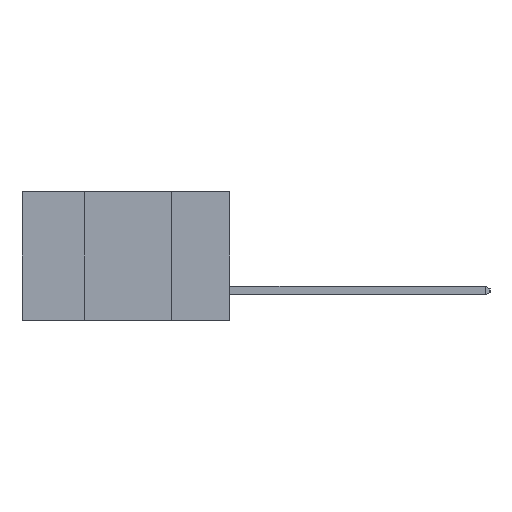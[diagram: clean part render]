
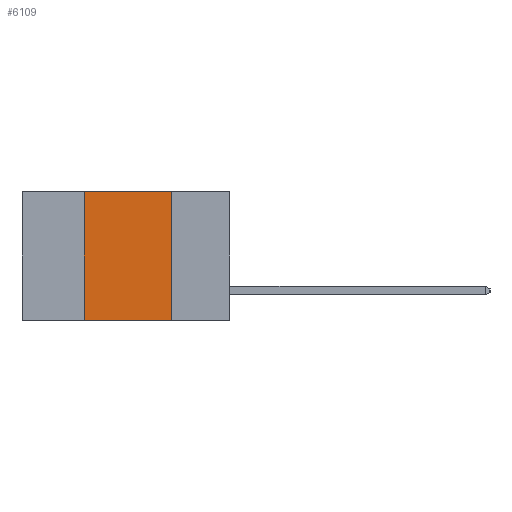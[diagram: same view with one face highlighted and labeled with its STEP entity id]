
A CAD part, left-side view. The second image highlights one B-rep face of the part: STEP entity #6109.
In plain terms, the highlighted planar face has unit normal (-1, 0, 0).
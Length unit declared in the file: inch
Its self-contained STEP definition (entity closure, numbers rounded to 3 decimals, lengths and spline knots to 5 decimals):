
#639 = CARTESIAN_POINT ( 'NONE',  ( 0., 0.6, -0.37 ) ) ;
#677 = LINE ( 'NONE', #12939, #9490 ) ;
#1038 = CARTESIAN_POINT ( 'NONE',  ( 0., 0.17, -0.37 ) ) ;
#1092 = LINE ( 'NONE', #10749, #21576 ) ;
#2657 = EDGE_CURVE ( 'NONE', #11655, #3269, #677, .T. ) ;
#3269 = VERTEX_POINT ( 'NONE', #16123 ) ;
#3472 = EDGE_CURVE ( 'NONE', #22373, #11655, #1092, .T. ) ;
#6109 = ADVANCED_FACE ( 'NONE', ( #21438 ), #7681, .F. ) ;
#6557 = VERTEX_POINT ( 'NONE', #1038 ) ;
#6902 = VECTOR ( 'NONE', #10671, 39.37008 ) ;
#7468 = ORIENTED_EDGE ( 'NONE', *, *, #3472, .F. ) ;
#7681 = PLANE ( 'NONE',  #22489 ) ;
#7974 = DIRECTION ( 'NONE',  ( 0., 0., 1. ) ) ;
#9490 = VECTOR ( 'NONE', #12769, 39.37008 ) ;
#9627 = DIRECTION ( 'NONE',  ( 0., 0., -1. ) ) ;
#10671 = DIRECTION ( 'NONE',  ( 0., -1., 0. ) ) ;
#10739 = EDGE_LOOP ( 'NONE', ( #23275, #14914, #7468, #23697 ) ) ;
#10749 = CARTESIAN_POINT ( 'NONE',  ( 0., 0.42, -0.37 ) ) ;
#11137 = CARTESIAN_POINT ( 'NONE',  ( 0., 0.42, 0. ) ) ;
#11655 = VERTEX_POINT ( 'NONE', #11137 ) ;
#11658 = DIRECTION ( 'NONE',  ( 0., 0., -1. ) ) ;
#12769 = DIRECTION ( 'NONE',  ( 0., -1., 0. ) ) ;
#12939 = CARTESIAN_POINT ( 'NONE',  ( 0., 0.6, 0. ) ) ;
#14914 = ORIENTED_EDGE ( 'NONE', *, *, #2657, .F. ) ;
#15738 = CARTESIAN_POINT ( 'NONE',  ( 0., 0.42, -0.37 ) ) ;
#16123 = CARTESIAN_POINT ( 'NONE',  ( 0., 0.17, 0. ) ) ;
#17741 = LINE ( 'NONE', #21420, #22908 ) ;
#18044 = LINE ( 'NONE', #639, #6902 ) ;
#21420 = CARTESIAN_POINT ( 'NONE',  ( 0., 0.17, -0.37 ) ) ;
#21438 = FACE_OUTER_BOUND ( 'NONE', #10739, .T. ) ;
#21448 = CARTESIAN_POINT ( 'NONE',  ( 0., 0.6, 0. ) ) ;
#21576 = VECTOR ( 'NONE', #7974, 39.37008 ) ;
#22373 = VERTEX_POINT ( 'NONE', #15738 ) ;
#22489 = AXIS2_PLACEMENT_3D ( 'NONE', #21448, #23407, #11658 ) ;
#22908 = VECTOR ( 'NONE', #9627, 39.37008 ) ;
#23275 = ORIENTED_EDGE ( 'NONE', *, *, #23614, .F. ) ;
#23407 = DIRECTION ( 'NONE',  ( 1., 0., 0. ) ) ;
#23614 = EDGE_CURVE ( 'NONE', #3269, #6557, #17741, .T. ) ;
#23697 = ORIENTED_EDGE ( 'NONE', *, *, #23853, .T. ) ;
#23853 = EDGE_CURVE ( 'NONE', #22373, #6557, #18044, .T. ) ;
